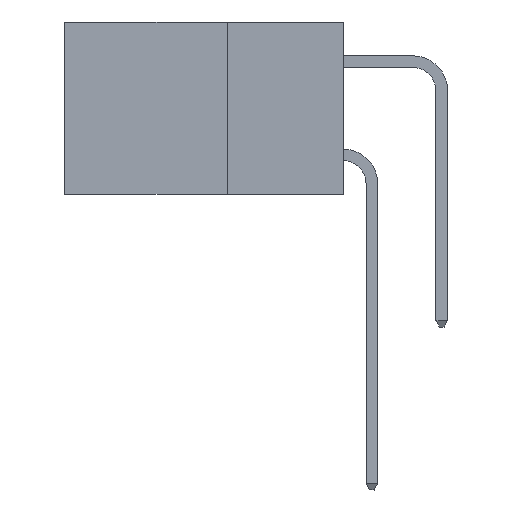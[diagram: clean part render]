
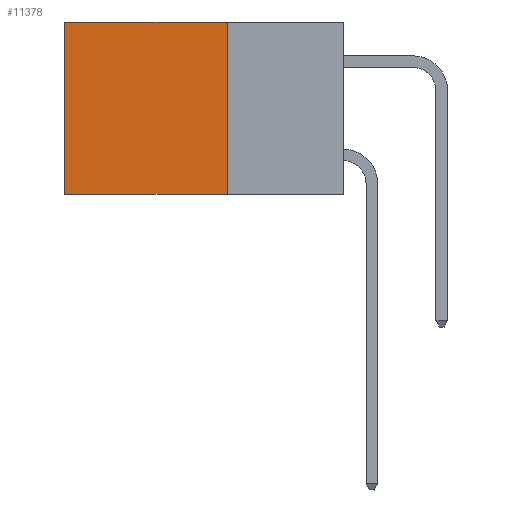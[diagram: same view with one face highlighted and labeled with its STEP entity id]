
A CAD part, left-side view. The second image highlights one B-rep face of the part: STEP entity #11378.
In plain terms, the highlighted planar face has unit normal (-1, 0, 0).
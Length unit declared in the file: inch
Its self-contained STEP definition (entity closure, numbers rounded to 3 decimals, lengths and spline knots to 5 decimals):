
#1654 = VECTOR ( 'NONE', #17967, 39.37008 ) ;
#2938 = EDGE_CURVE ( 'NONE', #6892, #6373, #23351, .T. ) ;
#3691 = DIRECTION ( 'NONE',  ( 0., 0., -1. ) ) ;
#3821 = VERTEX_POINT ( 'NONE', #21860 ) ;
#5057 = DIRECTION ( 'NONE',  ( 0., 0., -1. ) ) ;
#6266 = CARTESIAN_POINT ( 'NONE',  ( 0.298, 0.25, 0. ) ) ;
#6373 = VERTEX_POINT ( 'NONE', #12870 ) ;
#6756 = ORIENTED_EDGE ( 'NONE', *, *, #2938, .T. ) ;
#6825 = DIRECTION ( 'NONE',  ( 0., 1., 0. ) ) ;
#6837 = EDGE_CURVE ( 'NONE', #3821, #19544, #14086, .T. ) ;
#6892 = VERTEX_POINT ( 'NONE', #6266 ) ;
#7327 = CARTESIAN_POINT ( 'NONE',  ( 0.298, 0.25, -0.37 ) ) ;
#8284 = ORIENTED_EDGE ( 'NONE', *, *, #24586, .T. ) ;
#8547 = VECTOR ( 'NONE', #20025, 39.37008 ) ;
#8790 = ORIENTED_EDGE ( 'NONE', *, *, #23635, .F. ) ;
#8940 = VECTOR ( 'NONE', #6825, 39.37008 ) ;
#10640 = FACE_OUTER_BOUND ( 'NONE', #19783, .T. ) ;
#10895 = CARTESIAN_POINT ( 'NONE',  ( 0.298, 0.6, 0. ) ) ;
#11378 = ADVANCED_FACE ( 'NONE', ( #10640 ), #11497, .F. ) ;
#11497 = PLANE ( 'NONE',  #20554 ) ;
#12192 = CARTESIAN_POINT ( 'NONE',  ( 0.298, 0.25, 0. ) ) ;
#12870 = CARTESIAN_POINT ( 'NONE',  ( 0.298, 0.6, 0. ) ) ;
#13454 = CARTESIAN_POINT ( 'NONE',  ( 0.298, 0.25, 0. ) ) ;
#14086 = LINE ( 'NONE', #7327, #8940 ) ;
#15417 = DIRECTION ( 'NONE',  ( 1., 0., 0. ) ) ;
#15913 = CARTESIAN_POINT ( 'NONE',  ( 0.298, 0.6, -0.37 ) ) ;
#16793 = ORIENTED_EDGE ( 'NONE', *, *, #6837, .F. ) ;
#17967 = DIRECTION ( 'NONE',  ( 0., 0., -1. ) ) ;
#19544 = VERTEX_POINT ( 'NONE', #15913 ) ;
#19783 = EDGE_LOOP ( 'NONE', ( #8284, #16793, #8790, #6756 ) ) ;
#19913 = CARTESIAN_POINT ( 'NONE',  ( 0.298, 0.25, 0. ) ) ;
#20025 = DIRECTION ( 'NONE',  ( 0., 1., 0. ) ) ;
#20554 = AXIS2_PLACEMENT_3D ( 'NONE', #13454, #15417, #3691 ) ;
#20581 = LINE ( 'NONE', #10895, #25011 ) ;
#21860 = CARTESIAN_POINT ( 'NONE',  ( 0.298, 0.25, -0.37 ) ) ;
#22398 = LINE ( 'NONE', #12192, #1654 ) ;
#23351 = LINE ( 'NONE', #19913, #8547 ) ;
#23635 = EDGE_CURVE ( 'NONE', #6892, #3821, #22398, .T. ) ;
#24586 = EDGE_CURVE ( 'NONE', #6373, #19544, #20581, .T. ) ;
#25011 = VECTOR ( 'NONE', #5057, 39.37008 ) ;
